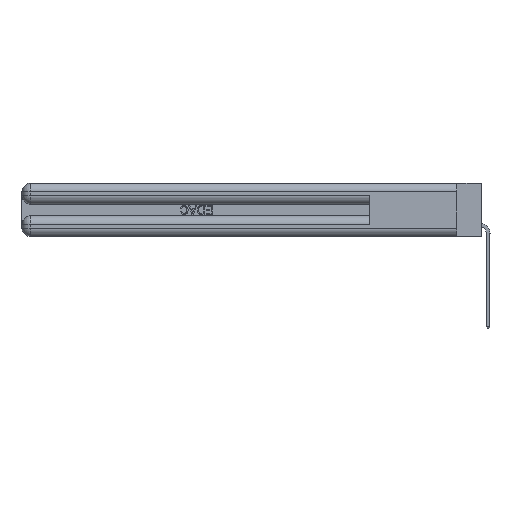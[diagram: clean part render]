
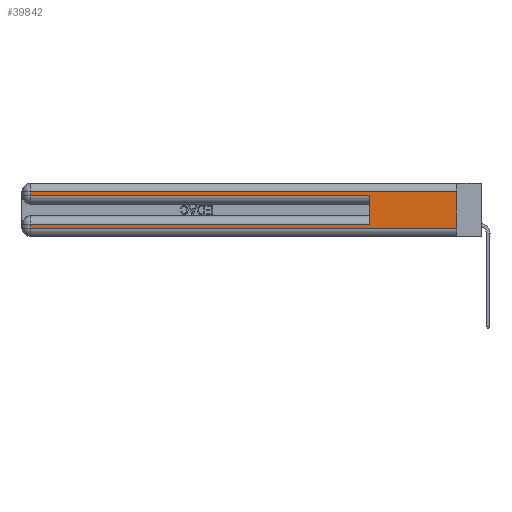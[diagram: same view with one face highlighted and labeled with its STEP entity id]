
A CAD part, left-side view. The second image highlights one B-rep face of the part: STEP entity #39842.
In plain terms, the highlighted planar face has unit normal (-1, 0, 0).
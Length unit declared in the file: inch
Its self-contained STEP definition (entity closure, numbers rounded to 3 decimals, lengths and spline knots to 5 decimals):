
#1639 = VECTOR ( 'NONE', #44789, 39.37008 ) ;
#1792 = EDGE_CURVE ( 'NONE', #35436, #5299, #6256, .T. ) ;
#1840 = DIRECTION ( 'NONE',  ( 0., -1., 0. ) ) ;
#3750 = VECTOR ( 'NONE', #43887, 39.37008 ) ;
#4926 = CARTESIAN_POINT ( 'NONE',  ( 0., 0., 0.31 ) ) ;
#5179 = EDGE_CURVE ( 'NONE', #33642, #27378, #45401, .T. ) ;
#5299 = VERTEX_POINT ( 'NONE', #20079 ) ;
#5808 = VERTEX_POINT ( 'NONE', #40638 ) ;
#5930 = LINE ( 'NONE', #32320, #23762 ) ;
#6256 = LINE ( 'NONE', #39645, #3750 ) ;
#6943 = PLANE ( 'NONE',  #30497 ) ;
#7184 = LINE ( 'NONE', #10106, #16619 ) ;
#7245 = CARTESIAN_POINT ( 'NONE',  ( 0., 0.6, 0.145 ) ) ;
#7418 = DIRECTION ( 'NONE',  ( 0., 0., 1. ) ) ;
#7987 = ORIENTED_EDGE ( 'NONE', *, *, #17453, .T. ) ;
#9002 = LINE ( 'NONE', #11102, #42011 ) ;
#10106 = CARTESIAN_POINT ( 'NONE',  ( 0., 0., 0.31 ) ) ;
#10302 = LINE ( 'NONE', #7245, #19840 ) ;
#11102 = CARTESIAN_POINT ( 'NONE',  ( 0., 0., 0.085 ) ) ;
#11103 = EDGE_CURVE ( 'NONE', #27378, #25667, #5930, .T. ) ;
#13070 = ORIENTED_EDGE ( 'NONE', *, *, #15161, .T. ) ;
#13197 = CARTESIAN_POINT ( 'NONE',  ( 0., 0., 0.37 ) ) ;
#13223 = VERTEX_POINT ( 'NONE', #4926 ) ;
#14269 = ORIENTED_EDGE ( 'NONE', *, *, #11103, .T. ) ;
#14357 = ORIENTED_EDGE ( 'NONE', *, *, #38098, .F. ) ;
#15161 = EDGE_CURVE ( 'NONE', #5299, #5808, #18148, .T. ) ;
#15235 = ORIENTED_EDGE ( 'NONE', *, *, #49982, .T. ) ;
#16619 = VECTOR ( 'NONE', #46655, 39.37008 ) ;
#17453 = EDGE_CURVE ( 'NONE', #13223, #33642, #7184, .T. ) ;
#18148 = LINE ( 'NONE', #49864, #31525 ) ;
#19840 = VECTOR ( 'NONE', #7418, 39.37008 ) ;
#19930 = CARTESIAN_POINT ( 'NONE',  ( 0., 2.94, 0.085 ) ) ;
#20079 = CARTESIAN_POINT ( 'NONE',  ( 0., 2.94, 0.06 ) ) ;
#23762 = VECTOR ( 'NONE', #40173, 39.37008 ) ;
#24656 = FACE_OUTER_BOUND ( 'NONE', #32983, .T. ) ;
#25667 = VERTEX_POINT ( 'NONE', #37843 ) ;
#26707 = VERTEX_POINT ( 'NONE', #47222 ) ;
#27378 = VERTEX_POINT ( 'NONE', #28276 ) ;
#28276 = CARTESIAN_POINT ( 'NONE',  ( 0., 2.94, 0.285 ) ) ;
#29214 = LINE ( 'NONE', #13197, #31204 ) ;
#30497 = AXIS2_PLACEMENT_3D ( 'NONE', #43296, #34776, #51230 ) ;
#31204 = VECTOR ( 'NONE', #52162, 39.37008 ) ;
#31525 = VECTOR ( 'NONE', #1840, 39.37008 ) ;
#32320 = CARTESIAN_POINT ( 'NONE',  ( 0., 0., 0.285 ) ) ;
#32661 = DIRECTION ( 'NONE',  ( 0., 1., 0. ) ) ;
#32983 = EDGE_LOOP ( 'NONE', ( #35503, #7987, #48834, #14269, #14357, #15235, #42159, #13070 ) ) ;
#33447 = EDGE_CURVE ( 'NONE', #13223, #5808, #29214, .T. ) ;
#33642 = VERTEX_POINT ( 'NONE', #47148 ) ;
#34776 = DIRECTION ( 'NONE',  ( 1., 0., 0. ) ) ;
#35436 = VERTEX_POINT ( 'NONE', #19930 ) ;
#35503 = ORIENTED_EDGE ( 'NONE', *, *, #33447, .F. ) ;
#37843 = CARTESIAN_POINT ( 'NONE',  ( 0., 0.6, 0.285 ) ) ;
#38098 = EDGE_CURVE ( 'NONE', #26707, #25667, #10302, .T. ) ;
#39645 = CARTESIAN_POINT ( 'NONE',  ( 0., 2.94, 0.37 ) ) ;
#39842 = ADVANCED_FACE ( 'NONE', ( #24656 ), #6943, .F. ) ;
#40173 = DIRECTION ( 'NONE',  ( 0., -1., 0. ) ) ;
#40638 = CARTESIAN_POINT ( 'NONE',  ( 0., 0., 0.06 ) ) ;
#42011 = VECTOR ( 'NONE', #32661, 39.37008 ) ;
#42159 = ORIENTED_EDGE ( 'NONE', *, *, #1792, .T. ) ;
#43296 = CARTESIAN_POINT ( 'NONE',  ( 0., 0., 0.37 ) ) ;
#43887 = DIRECTION ( 'NONE',  ( 0., 0., -1. ) ) ;
#44789 = DIRECTION ( 'NONE',  ( 0., 0., -1. ) ) ;
#45401 = LINE ( 'NONE', #49339, #1639 ) ;
#46655 = DIRECTION ( 'NONE',  ( 0., 1., 0. ) ) ;
#47148 = CARTESIAN_POINT ( 'NONE',  ( 0., 2.94, 0.31 ) ) ;
#47222 = CARTESIAN_POINT ( 'NONE',  ( 0., 0.6, 0.085 ) ) ;
#48834 = ORIENTED_EDGE ( 'NONE', *, *, #5179, .T. ) ;
#49339 = CARTESIAN_POINT ( 'NONE',  ( 0., 2.94, 0.37 ) ) ;
#49864 = CARTESIAN_POINT ( 'NONE',  ( 0., 0., 0.06 ) ) ;
#49982 = EDGE_CURVE ( 'NONE', #26707, #35436, #9002, .T. ) ;
#51230 = DIRECTION ( 'NONE',  ( 0., 0., -1. ) ) ;
#52162 = DIRECTION ( 'NONE',  ( 0., 0., -1. ) ) ;
